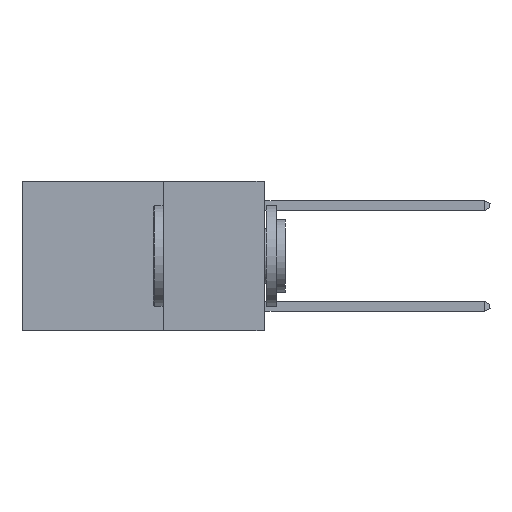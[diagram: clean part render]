
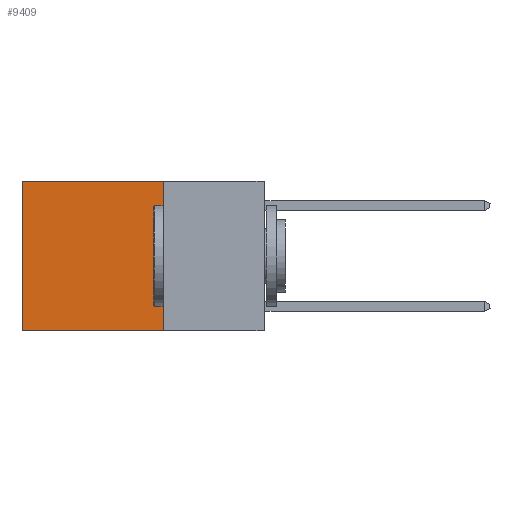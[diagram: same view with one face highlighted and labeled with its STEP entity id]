
A CAD part, left-side view. The second image highlights one B-rep face of the part: STEP entity #9409.
In plain terms, the highlighted planar face has unit normal (-1, 0, 0).
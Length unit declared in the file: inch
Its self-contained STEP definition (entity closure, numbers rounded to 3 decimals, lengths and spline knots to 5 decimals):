
#364 = CARTESIAN_POINT ( 'NONE',  ( 0.2625, 0.25, 0. ) ) ;
#705 = VECTOR ( 'NONE', #2047, 39.37008 ) ;
#1450 = CARTESIAN_POINT ( 'NONE',  ( 0.2625, 0.25, -0.37 ) ) ;
#1761 = AXIS2_PLACEMENT_3D ( 'NONE', #364, #4242, #7181 ) ;
#2047 = DIRECTION ( 'NONE',  ( 0., 1., 0. ) ) ;
#2102 = CARTESIAN_POINT ( 'NONE',  ( 0.2625, 0.6, -0.37 ) ) ;
#2338 = EDGE_CURVE ( 'NONE', #9832, #5893, #10650, .T. ) ;
#2934 = CARTESIAN_POINT ( 'NONE',  ( 0.2625, 0.25, 0. ) ) ;
#2937 = LINE ( 'NONE', #6979, #5821 ) ;
#3717 = DIRECTION ( 'NONE',  ( 0., 0., -1. ) ) ;
#4242 = DIRECTION ( 'NONE',  ( 1., 0., 0. ) ) ;
#5189 = FACE_OUTER_BOUND ( 'NONE', #9854, .T. ) ;
#5648 = ORIENTED_EDGE ( 'NONE', *, *, #8109, .T. ) ;
#5821 = VECTOR ( 'NONE', #11500, 39.37008 ) ;
#5893 = VERTEX_POINT ( 'NONE', #7862 ) ;
#6228 = EDGE_CURVE ( 'NONE', #9832, #10800, #11578, .T. ) ;
#6489 = DIRECTION ( 'NONE',  ( 0., 1., 0. ) ) ;
#6979 = CARTESIAN_POINT ( 'NONE',  ( 0.2625, 0.6, 0. ) ) ;
#6991 = CARTESIAN_POINT ( 'NONE',  ( 0.2625, 0.25, 0. ) ) ;
#7181 = DIRECTION ( 'NONE',  ( 0., 0., -1. ) ) ;
#7862 = CARTESIAN_POINT ( 'NONE',  ( 0.2625, 0.6, 0. ) ) ;
#8109 = EDGE_CURVE ( 'NONE', #5893, #8779, #2937, .T. ) ;
#8478 = CARTESIAN_POINT ( 'NONE',  ( 0.2625, 0.25, -0.37 ) ) ;
#8594 = VECTOR ( 'NONE', #6489, 39.37008 ) ;
#8779 = VERTEX_POINT ( 'NONE', #2102 ) ;
#8854 = ORIENTED_EDGE ( 'NONE', *, *, #6228, .F. ) ;
#8986 = PLANE ( 'NONE',  #1761 ) ;
#9389 = LINE ( 'NONE', #8478, #8594 ) ;
#9409 = ADVANCED_FACE ( 'NONE', ( #5189 ), #8986, .F. ) ;
#9832 = VERTEX_POINT ( 'NONE', #6991 ) ;
#9854 = EDGE_LOOP ( 'NONE', ( #5648, #11069, #8854, #10999 ) ) ;
#10650 = LINE ( 'NONE', #2934, #705 ) ;
#10659 = CARTESIAN_POINT ( 'NONE',  ( 0.2625, 0.25, 0. ) ) ;
#10738 = VECTOR ( 'NONE', #3717, 39.37008 ) ;
#10800 = VERTEX_POINT ( 'NONE', #1450 ) ;
#10999 = ORIENTED_EDGE ( 'NONE', *, *, #2338, .T. ) ;
#11042 = EDGE_CURVE ( 'NONE', #10800, #8779, #9389, .T. ) ;
#11069 = ORIENTED_EDGE ( 'NONE', *, *, #11042, .F. ) ;
#11500 = DIRECTION ( 'NONE',  ( 0., 0., -1. ) ) ;
#11578 = LINE ( 'NONE', #10659, #10738 ) ;
